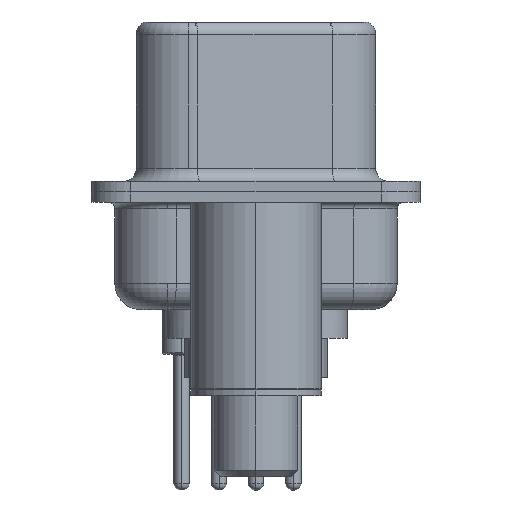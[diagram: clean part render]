
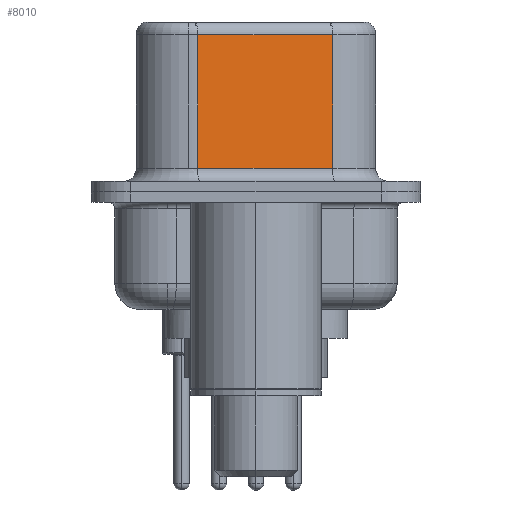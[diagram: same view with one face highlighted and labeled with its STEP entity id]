
A CAD part, left-side view. The second image highlights one B-rep face of the part: STEP entity #8010.
In plain terms, the highlighted planar face has unit normal (-0.985, -0.174, 0).
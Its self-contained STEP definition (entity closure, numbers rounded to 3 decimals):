
#1424 = ORIENTED_EDGE ( 'NONE', *, *, #17525, .T. ) ;
#1708 = PLANE ( 'NONE',  #20163 ) ;
#2365 = CARTESIAN_POINT ( 'NONE',  ( 4.58, -2.927, 6.52 ) ) ;
#2665 = LINE ( 'NONE', #11626, #11238 ) ;
#3325 = CARTESIAN_POINT ( 'NONE',  ( 4.58, -2.927, 6.52 ) ) ;
#3394 = DIRECTION ( 'NONE',  ( -0.174, 0.985, 0. ) ) ;
#3800 = VECTOR ( 'NONE', #16523, 1000. ) ;
#3999 = DIRECTION ( 'NONE',  ( 0., 0., -1. ) ) ;
#4128 = VERTEX_POINT ( 'NONE', #7470 ) ;
#4798 = LINE ( 'NONE', #14914, #3800 ) ;
#5112 = FACE_OUTER_BOUND ( 'NONE', #12996, .T. ) ;
#7470 = CARTESIAN_POINT ( 'NONE',  ( 3.67, 2.233, 0.9 ) ) ;
#8010 = ADVANCED_FACE ( 'NONE', ( #5112 ), #1708, .F. ) ;
#8061 = VERTEX_POINT ( 'NONE', #16412 ) ;
#9058 = VECTOR ( 'NONE', #3999, 1000. ) ;
#9584 = LINE ( 'NONE', #2365, #9058 ) ;
#10129 = CARTESIAN_POINT ( 'NONE',  ( 4.58, -2.927, 6.02 ) ) ;
#11009 = EDGE_CURVE ( 'NONE', #19230, #4128, #4798, .T. ) ;
#11238 = VECTOR ( 'NONE', #14929, 1000. ) ;
#11626 = CARTESIAN_POINT ( 'NONE',  ( 4.58, -2.927, 0.9 ) ) ;
#11812 = DIRECTION ( 'NONE',  ( -0.174, 0.985, 0. ) ) ;
#12303 = CARTESIAN_POINT ( 'NONE',  ( 3.67, 2.233, 6.02 ) ) ;
#12884 = ORIENTED_EDGE ( 'NONE', *, *, #19983, .F. ) ;
#12996 = EDGE_LOOP ( 'NONE', ( #12884, #13392, #13892, #1424 ) ) ;
#13095 = DIRECTION ( 'NONE',  ( 0.985, 0.174, 0. ) ) ;
#13392 = ORIENTED_EDGE ( 'NONE', *, *, #20621, .T. ) ;
#13892 = ORIENTED_EDGE ( 'NONE', *, *, #11009, .T. ) ;
#14295 = VERTEX_POINT ( 'NONE', #14346 ) ;
#14346 = CARTESIAN_POINT ( 'NONE',  ( 4.58, -2.927, 6.02 ) ) ;
#14914 = CARTESIAN_POINT ( 'NONE',  ( 3.67, 2.233, 6.52 ) ) ;
#14929 = DIRECTION ( 'NONE',  ( 0.174, -0.985, 0. ) ) ;
#16412 = CARTESIAN_POINT ( 'NONE',  ( 4.58, -2.927, 0.9 ) ) ;
#16523 = DIRECTION ( 'NONE',  ( 0., 0., -1. ) ) ;
#17525 = EDGE_CURVE ( 'NONE', #4128, #8061, #2665, .T. ) ;
#18026 = VECTOR ( 'NONE', #11812, 1000. ) ;
#18540 = LINE ( 'NONE', #10129, #18026 ) ;
#19230 = VERTEX_POINT ( 'NONE', #12303 ) ;
#19983 = EDGE_CURVE ( 'NONE', #14295, #8061, #9584, .T. ) ;
#20163 = AXIS2_PLACEMENT_3D ( 'NONE', #3325, #13095, #3394 ) ;
#20621 = EDGE_CURVE ( 'NONE', #14295, #19230, #18540, .T. ) ;
